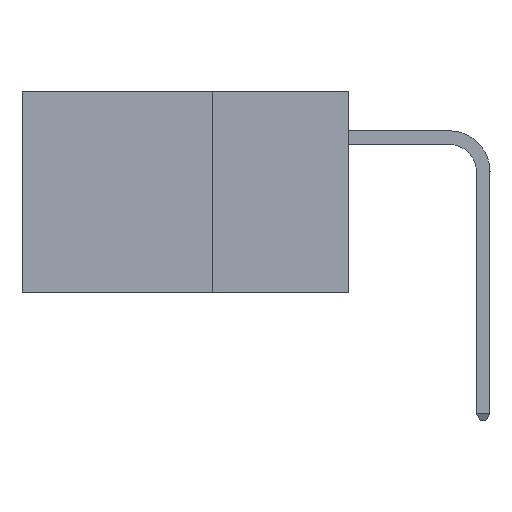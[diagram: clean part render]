
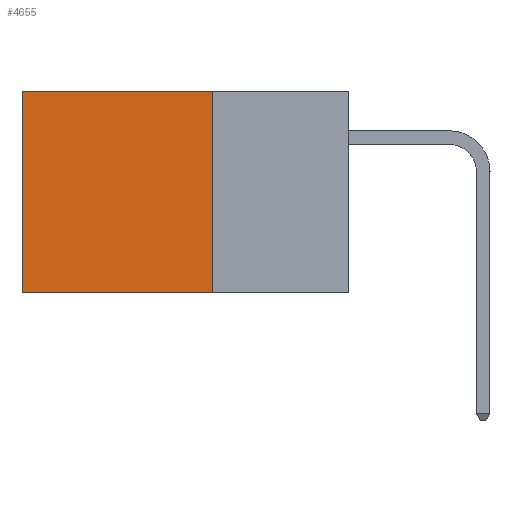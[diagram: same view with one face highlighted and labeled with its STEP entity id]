
A CAD part, left-side view. The second image highlights one B-rep face of the part: STEP entity #4655.
In plain terms, the highlighted planar face has unit normal (-1, 0, 0).
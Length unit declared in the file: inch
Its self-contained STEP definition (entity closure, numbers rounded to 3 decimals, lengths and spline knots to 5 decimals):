
#1529 = EDGE_CURVE ( 'NONE', #16547, #14201, #4602, .T. ) ;
#3486 = CARTESIAN_POINT ( 'NONE',  ( 0.2875, 0.25, -0.37 ) ) ;
#3533 = PLANE ( 'NONE',  #14092 ) ;
#4354 = CARTESIAN_POINT ( 'NONE',  ( 0.2875, 0.6, -0.37 ) ) ;
#4431 = EDGE_CURVE ( 'NONE', #13175, #6214, #15319, .T. ) ;
#4602 = LINE ( 'NONE', #21604, #17712 ) ;
#4655 = ADVANCED_FACE ( 'NONE', ( #18830 ), #3533, .F. ) ;
#5883 = CARTESIAN_POINT ( 'NONE',  ( 0.2875, 0.6, 0. ) ) ;
#6214 = VERTEX_POINT ( 'NONE', #4354 ) ;
#6559 = ORIENTED_EDGE ( 'NONE', *, *, #17010, .F. ) ;
#7847 = CARTESIAN_POINT ( 'NONE',  ( 0.2875, 0.25, 0. ) ) ;
#8205 = LINE ( 'NONE', #20872, #17955 ) ;
#8580 = EDGE_CURVE ( 'NONE', #14201, #6214, #8205, .T. ) ;
#10069 = ORIENTED_EDGE ( 'NONE', *, *, #8580, .T. ) ;
#10835 = DIRECTION ( 'NONE',  ( 0., 1., 0. ) ) ;
#10931 = VECTOR ( 'NONE', #12499, 39.37008 ) ;
#11191 = EDGE_LOOP ( 'NONE', ( #10069, #17394, #6559, #17550 ) ) ;
#12415 = CARTESIAN_POINT ( 'NONE',  ( 0.2875, 0.25, 0. ) ) ;
#12499 = DIRECTION ( 'NONE',  ( 0., 0., -1. ) ) ;
#12801 = DIRECTION ( 'NONE',  ( 0., 0., -1. ) ) ;
#13175 = VERTEX_POINT ( 'NONE', #3486 ) ;
#13997 = LINE ( 'NONE', #14028, #10931 ) ;
#14028 = CARTESIAN_POINT ( 'NONE',  ( 0.2875, 0.25, 0. ) ) ;
#14092 = AXIS2_PLACEMENT_3D ( 'NONE', #12415, #21645, #12801 ) ;
#14193 = VECTOR ( 'NONE', #19062, 39.37008 ) ;
#14201 = VERTEX_POINT ( 'NONE', #5883 ) ;
#15319 = LINE ( 'NONE', #15419, #14193 ) ;
#15419 = CARTESIAN_POINT ( 'NONE',  ( 0.2875, 0.25, -0.37 ) ) ;
#16547 = VERTEX_POINT ( 'NONE', #7847 ) ;
#17010 = EDGE_CURVE ( 'NONE', #16547, #13175, #13997, .T. ) ;
#17056 = DIRECTION ( 'NONE',  ( 0., 0., -1. ) ) ;
#17394 = ORIENTED_EDGE ( 'NONE', *, *, #4431, .F. ) ;
#17550 = ORIENTED_EDGE ( 'NONE', *, *, #1529, .T. ) ;
#17712 = VECTOR ( 'NONE', #10835, 39.37008 ) ;
#17955 = VECTOR ( 'NONE', #17056, 39.37008 ) ;
#18830 = FACE_OUTER_BOUND ( 'NONE', #11191, .T. ) ;
#19062 = DIRECTION ( 'NONE',  ( 0., 1., 0. ) ) ;
#20872 = CARTESIAN_POINT ( 'NONE',  ( 0.2875, 0.6, 0. ) ) ;
#21604 = CARTESIAN_POINT ( 'NONE',  ( 0.2875, 0.25, 0. ) ) ;
#21645 = DIRECTION ( 'NONE',  ( 1., 0., 0. ) ) ;
